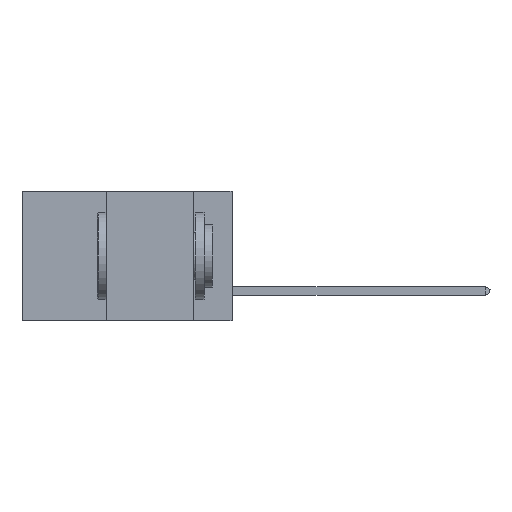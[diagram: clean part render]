
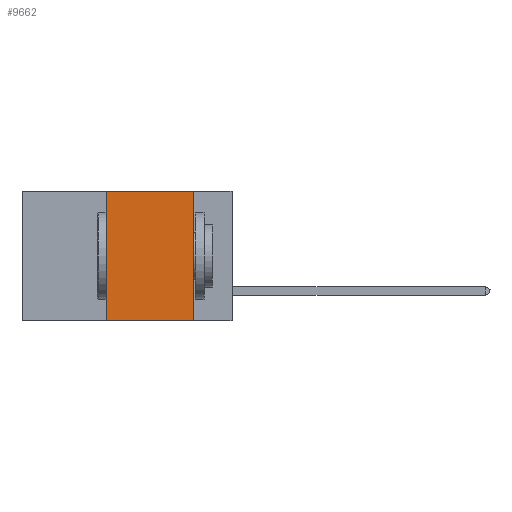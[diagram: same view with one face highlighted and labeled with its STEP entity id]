
A CAD part, left-side view. The second image highlights one B-rep face of the part: STEP entity #9662.
In plain terms, the highlighted planar face has unit normal (-1, 0, 0).
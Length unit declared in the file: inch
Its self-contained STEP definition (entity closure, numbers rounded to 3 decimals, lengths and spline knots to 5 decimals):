
#2 = DIRECTION ( 'NONE',  ( 0., 0., -1. ) ) ;
#1151 = FACE_OUTER_BOUND ( 'NONE', #19872, .T. ) ;
#1999 = DIRECTION ( 'NONE',  ( 0., 0., 1. ) ) ;
#2055 = ORIENTED_EDGE ( 'NONE', *, *, #16895, .F. ) ;
#3048 = EDGE_CURVE ( 'NONE', #6815, #17518, #11348, .T. ) ;
#3462 = CARTESIAN_POINT ( 'NONE',  ( 0., 0.6, 0. ) ) ;
#3827 = VERTEX_POINT ( 'NONE', #5448 ) ;
#4271 = DIRECTION ( 'NONE',  ( 0., 0., -1. ) ) ;
#4529 = CARTESIAN_POINT ( 'NONE',  ( 0., 0.6, -0.37 ) ) ;
#5448 = CARTESIAN_POINT ( 'NONE',  ( 0., 0.11, 0. ) ) ;
#6253 = LINE ( 'NONE', #4529, #12307 ) ;
#6815 = VERTEX_POINT ( 'NONE', #15773 ) ;
#6860 = LINE ( 'NONE', #11854, #14925 ) ;
#7340 = ORIENTED_EDGE ( 'NONE', *, *, #19433, .F. ) ;
#8454 = CARTESIAN_POINT ( 'NONE',  ( 0., 0.11, -0.37 ) ) ;
#8875 = VERTEX_POINT ( 'NONE', #8454 ) ;
#9662 = ADVANCED_FACE ( 'NONE', ( #1151 ), #12684, .F. ) ;
#10435 = ORIENTED_EDGE ( 'NONE', *, *, #11628, .T. ) ;
#10964 = CARTESIAN_POINT ( 'NONE',  ( 0., 0.36, 0. ) ) ;
#11348 = LINE ( 'NONE', #19546, #18884 ) ;
#11628 = EDGE_CURVE ( 'NONE', #6815, #8875, #6253, .T. ) ;
#11854 = CARTESIAN_POINT ( 'NONE',  ( 0., 0.11, 0. ) ) ;
#11866 = AXIS2_PLACEMENT_3D ( 'NONE', #12620, #15797, #2 ) ;
#12307 = VECTOR ( 'NONE', #14212, 39.37008 ) ;
#12620 = CARTESIAN_POINT ( 'NONE',  ( 0., 0.6, 0. ) ) ;
#12684 = PLANE ( 'NONE',  #11866 ) ;
#14212 = DIRECTION ( 'NONE',  ( 0., -1., 0. ) ) ;
#14846 = DIRECTION ( 'NONE',  ( 0., -1., 0. ) ) ;
#14925 = VECTOR ( 'NONE', #4271, 39.37008 ) ;
#15773 = CARTESIAN_POINT ( 'NONE',  ( 0., 0.36, -0.37 ) ) ;
#15797 = DIRECTION ( 'NONE',  ( 1., 0., 0. ) ) ;
#16568 = LINE ( 'NONE', #3462, #20280 ) ;
#16895 = EDGE_CURVE ( 'NONE', #17518, #3827, #16568, .T. ) ;
#17056 = ORIENTED_EDGE ( 'NONE', *, *, #3048, .F. ) ;
#17518 = VERTEX_POINT ( 'NONE', #10964 ) ;
#18884 = VECTOR ( 'NONE', #1999, 39.37008 ) ;
#19433 = EDGE_CURVE ( 'NONE', #3827, #8875, #6860, .T. ) ;
#19546 = CARTESIAN_POINT ( 'NONE',  ( 0., 0.36, 0. ) ) ;
#19872 = EDGE_LOOP ( 'NONE', ( #7340, #2055, #17056, #10435 ) ) ;
#20280 = VECTOR ( 'NONE', #14846, 39.37008 ) ;
